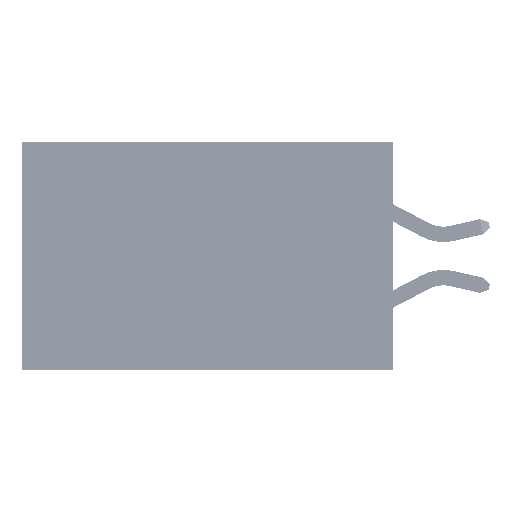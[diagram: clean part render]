
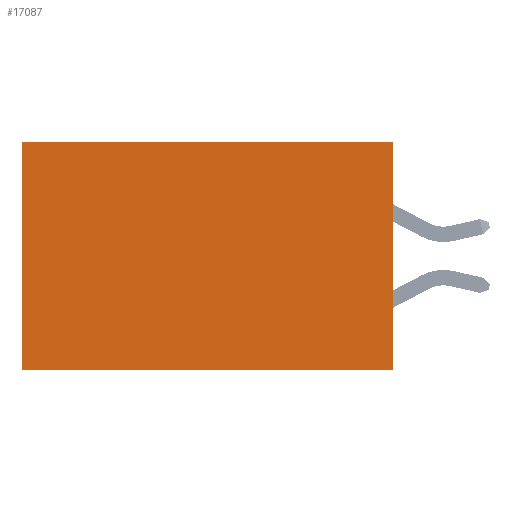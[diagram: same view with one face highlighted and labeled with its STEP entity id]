
A CAD part, left-side view. The second image highlights one B-rep face of the part: STEP entity #17087.
In plain terms, the highlighted planar face has unit normal (-1, 0, 0).
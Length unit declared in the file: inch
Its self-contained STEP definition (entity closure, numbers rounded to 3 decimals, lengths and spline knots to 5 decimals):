
#340 = EDGE_CURVE ( 'NONE', #27796, #6472, #15825, .T. ) ;
#2469 = EDGE_CURVE ( 'NONE', #9742, #27796, #18243, .T. ) ;
#5407 = LINE ( 'NONE', #28743, #5974 ) ;
#5974 = VECTOR ( 'NONE', #20968, 39.37008 ) ;
#6472 = VERTEX_POINT ( 'NONE', #20048 ) ;
#7766 = VECTOR ( 'NONE', #21626, 39.37008 ) ;
#9742 = VERTEX_POINT ( 'NONE', #30055 ) ;
#9747 = CARTESIAN_POINT ( 'NONE',  ( 0.2875, 0., 0. ) ) ;
#10334 = CARTESIAN_POINT ( 'NONE',  ( 0.2875, 0.6, 0. ) ) ;
#12115 = DIRECTION ( 'NONE',  ( 1., 0., 0. ) ) ;
#12178 = CARTESIAN_POINT ( 'NONE',  ( 0.2875, 0., -0.37 ) ) ;
#12770 = VECTOR ( 'NONE', #33613, 39.37008 ) ;
#15798 = AXIS2_PLACEMENT_3D ( 'NONE', #39730, #12115, #20029 ) ;
#15825 = LINE ( 'NONE', #10334, #12770 ) ;
#16996 = ORIENTED_EDGE ( 'NONE', *, *, #2469, .T. ) ;
#17087 = ADVANCED_FACE ( 'NONE', ( #35958 ), #19367, .F. ) ;
#18243 = LINE ( 'NONE', #9747, #7766 ) ;
#19367 = PLANE ( 'NONE',  #15798 ) ;
#20029 = DIRECTION ( 'NONE',  ( 0., 0., -1. ) ) ;
#20035 = EDGE_CURVE ( 'NONE', #9742, #42061, #30687, .T. ) ;
#20048 = CARTESIAN_POINT ( 'NONE',  ( 0.2875, 0.6, -0.37 ) ) ;
#20968 = DIRECTION ( 'NONE',  ( 0., 1., 0. ) ) ;
#21626 = DIRECTION ( 'NONE',  ( 0., 1., 0. ) ) ;
#22624 = ORIENTED_EDGE ( 'NONE', *, *, #20035, .F. ) ;
#26013 = CARTESIAN_POINT ( 'NONE',  ( 0.2875, 0., 0. ) ) ;
#27235 = EDGE_CURVE ( 'NONE', #42061, #6472, #5407, .T. ) ;
#27796 = VERTEX_POINT ( 'NONE', #40115 ) ;
#28743 = CARTESIAN_POINT ( 'NONE',  ( 0.2875, 0., -0.37 ) ) ;
#30055 = CARTESIAN_POINT ( 'NONE',  ( 0.2875, 0., 0. ) ) ;
#30687 = LINE ( 'NONE', #26013, #47333 ) ;
#31197 = ORIENTED_EDGE ( 'NONE', *, *, #340, .T. ) ;
#33613 = DIRECTION ( 'NONE',  ( 0., 0., -1. ) ) ;
#35958 = FACE_OUTER_BOUND ( 'NONE', #38206, .T. ) ;
#38206 = EDGE_LOOP ( 'NONE', ( #31197, #39311, #22624, #16996 ) ) ;
#39311 = ORIENTED_EDGE ( 'NONE', *, *, #27235, .F. ) ;
#39730 = CARTESIAN_POINT ( 'NONE',  ( 0.2875, 0., 0. ) ) ;
#40115 = CARTESIAN_POINT ( 'NONE',  ( 0.2875, 0.6, 0. ) ) ;
#42061 = VERTEX_POINT ( 'NONE', #12178 ) ;
#47333 = VECTOR ( 'NONE', #49703, 39.37008 ) ;
#49703 = DIRECTION ( 'NONE',  ( 0., 0., -1. ) ) ;
